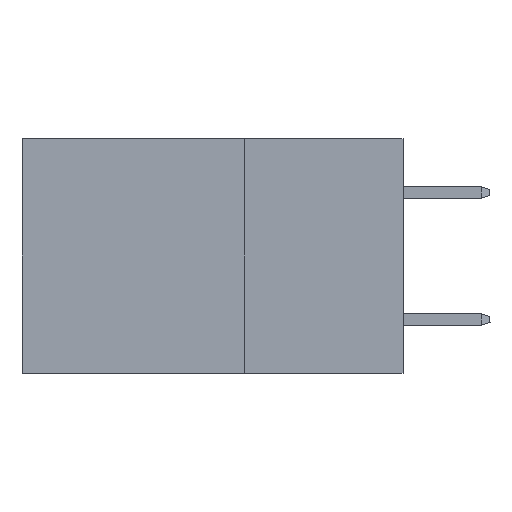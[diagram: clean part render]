
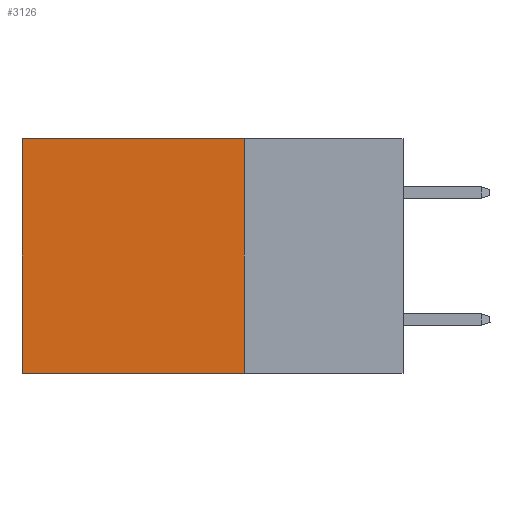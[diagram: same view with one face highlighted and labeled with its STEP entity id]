
A CAD part, left-side view. The second image highlights one B-rep face of the part: STEP entity #3126.
In plain terms, the highlighted planar face has unit normal (-1, 0, 0).
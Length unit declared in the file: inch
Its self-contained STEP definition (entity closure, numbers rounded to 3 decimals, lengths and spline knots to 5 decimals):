
#1861 = DIRECTION ( 'NONE',  ( 0., 1., 0. ) ) ;
#3100 = CARTESIAN_POINT ( 'NONE',  ( 0.2875, 0.25, -0.37 ) ) ;
#3126 = ADVANCED_FACE ( 'NONE', ( #16174 ), #3220, .F. ) ;
#3220 = PLANE ( 'NONE',  #18949 ) ;
#3240 = EDGE_LOOP ( 'NONE', ( #26487, #9987, #23971, #9393 ) ) ;
#3757 = VERTEX_POINT ( 'NONE', #10683 ) ;
#3875 = CARTESIAN_POINT ( 'NONE',  ( 0.2875, 0.6, 0. ) ) ;
#8212 = CARTESIAN_POINT ( 'NONE',  ( 0.2875, 0.25, 0. ) ) ;
#8490 = LINE ( 'NONE', #8212, #9247 ) ;
#9247 = VECTOR ( 'NONE', #1861, 39.37008 ) ;
#9393 = ORIENTED_EDGE ( 'NONE', *, *, #12467, .T. ) ;
#9987 = ORIENTED_EDGE ( 'NONE', *, *, #14612, .F. ) ;
#10683 = CARTESIAN_POINT ( 'NONE',  ( 0.2875, 0.6, -0.37 ) ) ;
#11756 = LINE ( 'NONE', #3100, #24571 ) ;
#11912 = EDGE_CURVE ( 'NONE', #16720, #22506, #15155, .T. ) ;
#12024 = CARTESIAN_POINT ( 'NONE',  ( 0.2875, 0.25, 0. ) ) ;
#12467 = EDGE_CURVE ( 'NONE', #16720, #25799, #8490, .T. ) ;
#12876 = DIRECTION ( 'NONE',  ( 1., 0., 0. ) ) ;
#12961 = LINE ( 'NONE', #3875, #26385 ) ;
#13105 = DIRECTION ( 'NONE',  ( 0., 0., -1. ) ) ;
#13135 = DIRECTION ( 'NONE',  ( 0., 0., -1. ) ) ;
#13701 = CARTESIAN_POINT ( 'NONE',  ( 0.2875, 0.25, 0. ) ) ;
#13865 = EDGE_CURVE ( 'NONE', #25799, #3757, #12961, .T. ) ;
#14612 = EDGE_CURVE ( 'NONE', #22506, #3757, #11756, .T. ) ;
#15155 = LINE ( 'NONE', #25852, #16434 ) ;
#15924 = DIRECTION ( 'NONE',  ( 0., 1., 0. ) ) ;
#16174 = FACE_OUTER_BOUND ( 'NONE', #3240, .T. ) ;
#16434 = VECTOR ( 'NONE', #13135, 39.37008 ) ;
#16720 = VERTEX_POINT ( 'NONE', #13701 ) ;
#17178 = DIRECTION ( 'NONE',  ( 0., 0., -1. ) ) ;
#18949 = AXIS2_PLACEMENT_3D ( 'NONE', #12024, #12876, #17178 ) ;
#22469 = CARTESIAN_POINT ( 'NONE',  ( 0.2875, 0.25, -0.37 ) ) ;
#22506 = VERTEX_POINT ( 'NONE', #22469 ) ;
#23971 = ORIENTED_EDGE ( 'NONE', *, *, #11912, .F. ) ;
#24571 = VECTOR ( 'NONE', #15924, 39.37008 ) ;
#25388 = CARTESIAN_POINT ( 'NONE',  ( 0.2875, 0.6, 0. ) ) ;
#25799 = VERTEX_POINT ( 'NONE', #25388 ) ;
#25852 = CARTESIAN_POINT ( 'NONE',  ( 0.2875, 0.25, 0. ) ) ;
#26385 = VECTOR ( 'NONE', #13105, 39.37008 ) ;
#26487 = ORIENTED_EDGE ( 'NONE', *, *, #13865, .T. ) ;
